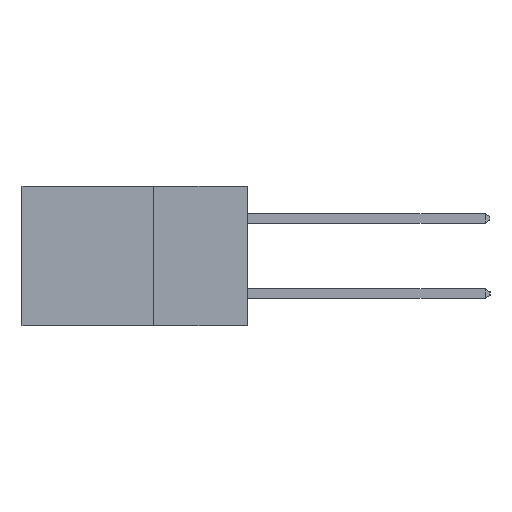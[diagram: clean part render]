
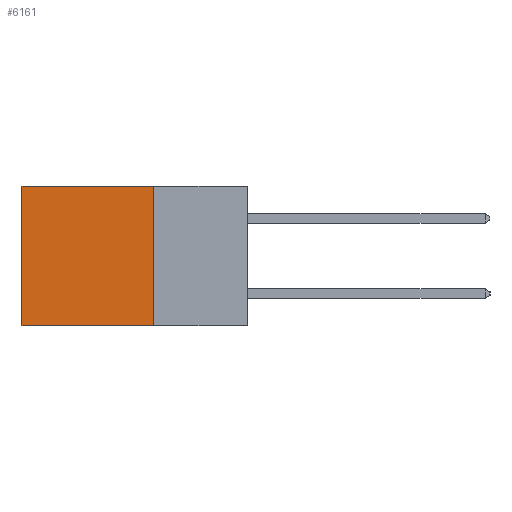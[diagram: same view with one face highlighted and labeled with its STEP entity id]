
A CAD part, left-side view. The second image highlights one B-rep face of the part: STEP entity #6161.
In plain terms, the highlighted planar face has unit normal (-1, 0, 0).
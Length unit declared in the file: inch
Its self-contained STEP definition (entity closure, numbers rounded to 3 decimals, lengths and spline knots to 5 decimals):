
#467 = DIRECTION ( 'NONE',  ( 0., 1., 0. ) ) ;
#1356 = VERTEX_POINT ( 'NONE', #7285 ) ;
#1510 = LINE ( 'NONE', #10567, #19131 ) ;
#2414 = ORIENTED_EDGE ( 'NONE', *, *, #19743, .T. ) ;
#2612 = CARTESIAN_POINT ( 'NONE',  ( 0.2615, 0.6, 0. ) ) ;
#3909 = ORIENTED_EDGE ( 'NONE', *, *, #8342, .F. ) ;
#4244 = VECTOR ( 'NONE', #12308, 39.37008 ) ;
#4640 = EDGE_CURVE ( 'NONE', #18561, #7838, #17841, .T. ) ;
#5171 = CARTESIAN_POINT ( 'NONE',  ( 0.2615, 0.25, -0.37 ) ) ;
#5665 = CARTESIAN_POINT ( 'NONE',  ( 0.2615, 0.25, -0.37 ) ) ;
#6026 = ORIENTED_EDGE ( 'NONE', *, *, #4640, .T. ) ;
#6161 = ADVANCED_FACE ( 'NONE', ( #9383 ), #9365, .F. ) ;
#6616 = LINE ( 'NONE', #22025, #15189 ) ;
#7285 = CARTESIAN_POINT ( 'NONE',  ( 0.2615, 0.25, 0. ) ) ;
#7838 = VERTEX_POINT ( 'NONE', #21402 ) ;
#8342 = EDGE_CURVE ( 'NONE', #1356, #18960, #19281, .T. ) ;
#8373 = ORIENTED_EDGE ( 'NONE', *, *, #10119, .F. ) ;
#9203 = DIRECTION ( 'NONE',  ( 0., 0., -1. ) ) ;
#9232 = DIRECTION ( 'NONE',  ( 1., 0., 0. ) ) ;
#9249 = CARTESIAN_POINT ( 'NONE',  ( 0.2615, 0.25, -0.37 ) ) ;
#9365 = PLANE ( 'NONE',  #9963 ) ;
#9383 = FACE_OUTER_BOUND ( 'NONE', #21569, .T. ) ;
#9963 = AXIS2_PLACEMENT_3D ( 'NONE', #9249, #9232, #9203 ) ;
#10119 = EDGE_CURVE ( 'NONE', #18960, #7838, #6616, .T. ) ;
#10567 = CARTESIAN_POINT ( 'NONE',  ( 0.2615, 0.25, 0. ) ) ;
#12308 = DIRECTION ( 'NONE',  ( 0., 0., -1. ) ) ;
#12495 = CARTESIAN_POINT ( 'NONE',  ( 0.2615, 0.6, -0.37 ) ) ;
#15189 = VECTOR ( 'NONE', #15283, 39.37008 ) ;
#15283 = DIRECTION ( 'NONE',  ( 0., 1., 0. ) ) ;
#15909 = DIRECTION ( 'NONE',  ( 0., 0., -1. ) ) ;
#17841 = LINE ( 'NONE', #12495, #4244 ) ;
#18561 = VERTEX_POINT ( 'NONE', #2612 ) ;
#18751 = VECTOR ( 'NONE', #15909, 39.37008 ) ;
#18960 = VERTEX_POINT ( 'NONE', #5171 ) ;
#19131 = VECTOR ( 'NONE', #467, 39.37008 ) ;
#19281 = LINE ( 'NONE', #5665, #18751 ) ;
#19743 = EDGE_CURVE ( 'NONE', #1356, #18561, #1510, .T. ) ;
#21402 = CARTESIAN_POINT ( 'NONE',  ( 0.2615, 0.6, -0.37 ) ) ;
#21569 = EDGE_LOOP ( 'NONE', ( #6026, #8373, #3909, #2414 ) ) ;
#22025 = CARTESIAN_POINT ( 'NONE',  ( 0.2615, 0.25, -0.37 ) ) ;
